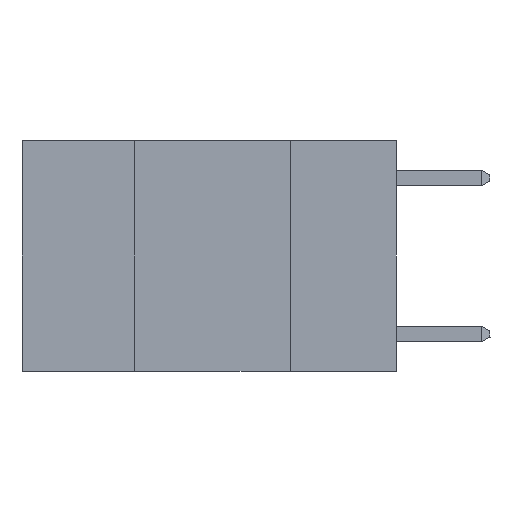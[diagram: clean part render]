
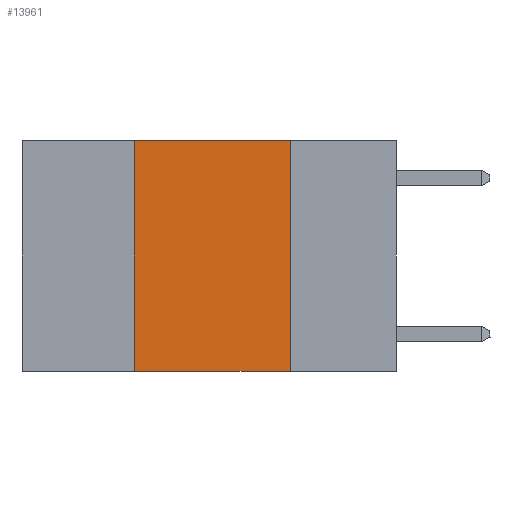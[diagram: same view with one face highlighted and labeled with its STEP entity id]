
A CAD part, left-side view. The second image highlights one B-rep face of the part: STEP entity #13961.
In plain terms, the highlighted planar face has unit normal (-1, 0, 0).
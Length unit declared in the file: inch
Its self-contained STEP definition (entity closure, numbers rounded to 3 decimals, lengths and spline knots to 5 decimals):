
#27 = LINE ( 'NONE', #18844, #221 ) ;
#221 = VECTOR ( 'NONE', #15852, 39.37008 ) ;
#355 = CARTESIAN_POINT ( 'NONE',  ( 0., 0.6, 0. ) ) ;
#1023 = ORIENTED_EDGE ( 'NONE', *, *, #4862, .F. ) ;
#1168 = ORIENTED_EDGE ( 'NONE', *, *, #15302, .T. ) ;
#2054 = VERTEX_POINT ( 'NONE', #9780 ) ;
#2094 = PLANE ( 'NONE',  #7746 ) ;
#3809 = DIRECTION ( 'NONE',  ( 1., 0., 0. ) ) ;
#3899 = VERTEX_POINT ( 'NONE', #6015 ) ;
#4100 = VECTOR ( 'NONE', #14515, 39.37008 ) ;
#4105 = LINE ( 'NONE', #13061, #4100 ) ;
#4709 = VERTEX_POINT ( 'NONE', #16880 ) ;
#4862 = EDGE_CURVE ( 'NONE', #4709, #5645, #15753, .T. ) ;
#5279 = CARTESIAN_POINT ( 'NONE',  ( 0., 0.42, 0. ) ) ;
#5645 = VERTEX_POINT ( 'NONE', #18314 ) ;
#6015 = CARTESIAN_POINT ( 'NONE',  ( 0., 0.17, 0. ) ) ;
#7658 = EDGE_CURVE ( 'NONE', #5645, #3899, #11376, .T. ) ;
#7746 = AXIS2_PLACEMENT_3D ( 'NONE', #355, #3809, #14816 ) ;
#9380 = FACE_OUTER_BOUND ( 'NONE', #18017, .T. ) ;
#9780 = CARTESIAN_POINT ( 'NONE',  ( 0., 0.17, -0.37 ) ) ;
#10398 = CARTESIAN_POINT ( 'NONE',  ( 0., 0.6, 0. ) ) ;
#11376 = LINE ( 'NONE', #10398, #11468 ) ;
#11468 = VECTOR ( 'NONE', #18045, 39.37008 ) ;
#13061 = CARTESIAN_POINT ( 'NONE',  ( 0., 0.6, -0.37 ) ) ;
#13961 = ADVANCED_FACE ( 'NONE', ( #9380 ), #2094, .F. ) ;
#14515 = DIRECTION ( 'NONE',  ( 0., -1., 0. ) ) ;
#14816 = DIRECTION ( 'NONE',  ( 0., 0., -1. ) ) ;
#15302 = EDGE_CURVE ( 'NONE', #4709, #2054, #4105, .T. ) ;
#15462 = VECTOR ( 'NONE', #19147, 39.37008 ) ;
#15753 = LINE ( 'NONE', #5279, #15462 ) ;
#15852 = DIRECTION ( 'NONE',  ( 0., 0., -1. ) ) ;
#16880 = CARTESIAN_POINT ( 'NONE',  ( 0., 0.42, -0.37 ) ) ;
#17883 = EDGE_CURVE ( 'NONE', #3899, #2054, #27, .T. ) ;
#18017 = EDGE_LOOP ( 'NONE', ( #19862, #19896, #1023, #1168 ) ) ;
#18045 = DIRECTION ( 'NONE',  ( 0., -1., 0. ) ) ;
#18314 = CARTESIAN_POINT ( 'NONE',  ( 0., 0.42, 0. ) ) ;
#18844 = CARTESIAN_POINT ( 'NONE',  ( 0., 0.17, 0. ) ) ;
#19147 = DIRECTION ( 'NONE',  ( 0., 0., 1. ) ) ;
#19862 = ORIENTED_EDGE ( 'NONE', *, *, #17883, .F. ) ;
#19896 = ORIENTED_EDGE ( 'NONE', *, *, #7658, .F. ) ;
